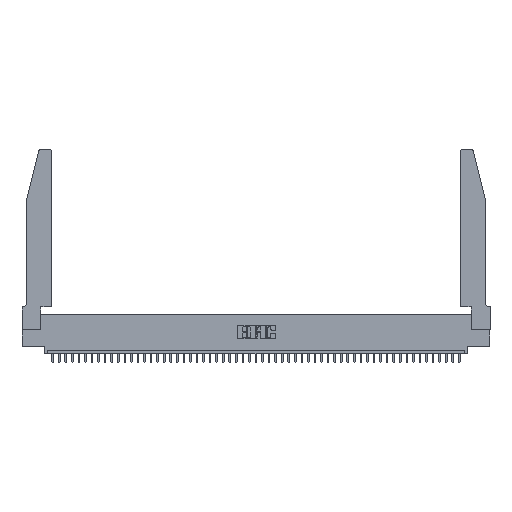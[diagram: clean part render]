
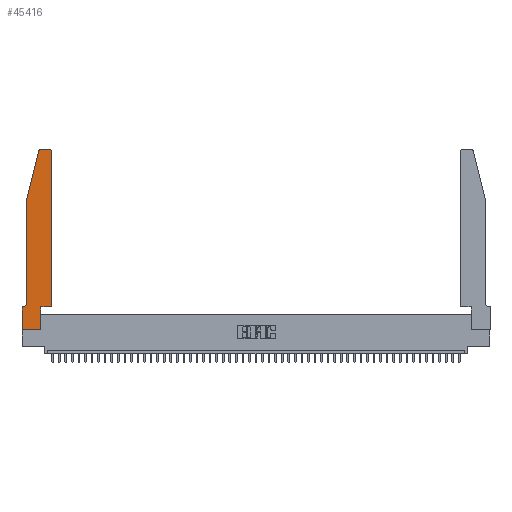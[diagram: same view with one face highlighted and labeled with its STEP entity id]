
A CAD part, top view. The second image highlights one B-rep face of the part: STEP entity #45416.
In plain terms, the highlighted planar face has unit normal (0, 0, 1).
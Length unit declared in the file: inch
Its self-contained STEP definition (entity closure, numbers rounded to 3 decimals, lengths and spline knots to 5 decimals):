
#341 = PLANE ( 'NONE',  #30279 ) ;
#1431 = LINE ( 'NONE', #37344, #19328 ) ;
#1948 = VERTEX_POINT ( 'NONE', #45646 ) ;
#2247 = ORIENTED_EDGE ( 'NONE', *, *, #24732, .T. ) ;
#2251 = DIRECTION ( 'NONE',  ( -1., 0., 0. ) ) ;
#2310 = CARTESIAN_POINT ( 'NONE',  ( 0.284, 2.72, 0.37 ) ) ;
#2726 = VECTOR ( 'NONE', #29254, 39.37008 ) ;
#3358 = AXIS2_PLACEMENT_3D ( 'NONE', #44362, #21430, #2251 ) ;
#3951 = LINE ( 'NONE', #23775, #9359 ) ;
#4026 = CARTESIAN_POINT ( 'NONE',  ( 0., 0.35, 0.37 ) ) ;
#4238 = ORIENTED_EDGE ( 'NONE', *, *, #40683, .T. ) ;
#6506 = VECTOR ( 'NONE', #29017, 39.37008 ) ;
#6556 = LINE ( 'NONE', #21689, #44270 ) ;
#6789 = CARTESIAN_POINT ( 'NONE',  ( 0.2865, 0.35, 0.37 ) ) ;
#6815 = CARTESIAN_POINT ( 'NONE',  ( 0., 0., 0.37 ) ) ;
#7213 = VERTEX_POINT ( 'NONE', #27663 ) ;
#8018 = LINE ( 'NONE', #9886, #2726 ) ;
#9359 = VECTOR ( 'NONE', #40073, 39.37008 ) ;
#9886 = CARTESIAN_POINT ( 'NONE',  ( 0.2865, 0.35, 0.37 ) ) ;
#10471 = DIRECTION ( 'NONE',  ( 1., 0., 0. ) ) ;
#10653 = LINE ( 'NONE', #16750, #6506 ) ;
#10890 = VERTEX_POINT ( 'NONE', #46269 ) ;
#11390 = EDGE_CURVE ( 'NONE', #10890, #7213, #33859, .T. ) ;
#11550 = DIRECTION ( 'NONE',  ( 0., 0., 1. ) ) ;
#11642 = DIRECTION ( 'NONE',  ( 0., 1., 0. ) ) ;
#11790 = EDGE_CURVE ( 'NONE', #43213, #23898, #8018, .T. ) ;
#13609 = VERTEX_POINT ( 'NONE', #44633 ) ;
#13889 = CARTESIAN_POINT ( 'NONE',  ( 0.4205, 2.72, 0.37 ) ) ;
#14196 = ORIENTED_EDGE ( 'NONE', *, *, #23156, .T. ) ;
#15186 = VERTEX_POINT ( 'NONE', #43532 ) ;
#15848 = DIRECTION ( 'NONE',  ( 1., 0., 0. ) ) ;
#15994 = AXIS2_PLACEMENT_3D ( 'NONE', #2310, #32896, #10471 ) ;
#16124 = CARTESIAN_POINT ( 'NONE',  ( 0.0755, 0.42, 0.37 ) ) ;
#16750 = CARTESIAN_POINT ( 'NONE',  ( 0., 0., 0.37 ) ) ;
#16976 = CARTESIAN_POINT ( 'NONE',  ( 0., 0.35, 0.37 ) ) ;
#17239 = EDGE_CURVE ( 'NONE', #40031, #40582, #37702, .T. ) ;
#17250 = EDGE_CURVE ( 'NONE', #15186, #34043, #18529, .T. ) ;
#17297 = LINE ( 'NONE', #45942, #26267 ) ;
#18529 = LINE ( 'NONE', #39431, #23836 ) ;
#19328 = VECTOR ( 'NONE', #41161, 39.37008 ) ;
#20838 = DIRECTION ( 'NONE',  ( 0., 0., 1. ) ) ;
#21008 = ORIENTED_EDGE ( 'NONE', *, *, #23446, .T. ) ;
#21430 = DIRECTION ( 'NONE',  ( 0., 0., -1. ) ) ;
#21513 = DIRECTION ( 'NONE',  ( 0., -1., 0. ) ) ;
#21606 = EDGE_CURVE ( 'NONE', #13609, #25990, #25603, .T. ) ;
#21689 = CARTESIAN_POINT ( 'NONE',  ( 0.2605, 2.75, 0.37 ) ) ;
#23156 = EDGE_CURVE ( 'NONE', #23898, #24640, #3951, .T. ) ;
#23446 = EDGE_CURVE ( 'NONE', #34043, #40031, #29663, .T. ) ;
#23775 = CARTESIAN_POINT ( 'NONE',  ( 0.4505, 0.35, 0.37 ) ) ;
#23836 = VECTOR ( 'NONE', #36988, 39.37008 ) ;
#23898 = VERTEX_POINT ( 'NONE', #6789 ) ;
#24589 = FACE_OUTER_BOUND ( 'NONE', #31035, .T. ) ;
#24640 = VERTEX_POINT ( 'NONE', #45241 ) ;
#24732 = EDGE_CURVE ( 'NONE', #25990, #15186, #1431, .T. ) ;
#24985 = LINE ( 'NONE', #6815, #25575 ) ;
#25575 = VECTOR ( 'NONE', #21513, 39.37008 ) ;
#25603 = CIRCLE ( 'NONE', #15994, 0.03 ) ;
#25990 = VERTEX_POINT ( 'NONE', #43515 ) ;
#26164 = ORIENTED_EDGE ( 'NONE', *, *, #11390, .T. ) ;
#26267 = VECTOR ( 'NONE', #11642, 39.37008 ) ;
#26702 = ORIENTED_EDGE ( 'NONE', *, *, #41178, .T. ) ;
#26908 = ORIENTED_EDGE ( 'NONE', *, *, #17250, .T. ) ;
#27663 = CARTESIAN_POINT ( 'NONE',  ( 0.4205, 2.75, 0.37 ) ) ;
#29017 = DIRECTION ( 'NONE',  ( 1., 0., 0. ) ) ;
#29254 = DIRECTION ( 'NONE',  ( 0., 1., 0. ) ) ;
#29392 = ORIENTED_EDGE ( 'NONE', *, *, #21606, .T. ) ;
#29663 = CIRCLE ( 'NONE', #3358, 0.07 ) ;
#30279 = AXIS2_PLACEMENT_3D ( 'NONE', #4026, #11550, #15848 ) ;
#31035 = EDGE_LOOP ( 'NONE', ( #4238, #29392, #2247, #26908, #21008, #43499, #39993, #26702, #38931, #14196, #33309, #26164 ) ) ;
#31607 = VECTOR ( 'NONE', #32754, 39.37008 ) ;
#32754 = DIRECTION ( 'NONE',  ( -1., 0., 0. ) ) ;
#32896 = DIRECTION ( 'NONE',  ( 0., 0., 1. ) ) ;
#33062 = CARTESIAN_POINT ( 'NONE',  ( 0.0055, 0.35, 0.37 ) ) ;
#33309 = ORIENTED_EDGE ( 'NONE', *, *, #40378, .T. ) ;
#33479 = AXIS2_PLACEMENT_3D ( 'NONE', #13889, #20838, #46283 ) ;
#33859 = CIRCLE ( 'NONE', #33479, 0.03 ) ;
#34043 = VERTEX_POINT ( 'NONE', #16124 ) ;
#36382 = CARTESIAN_POINT ( 'NONE',  ( 0.2865, 0., 0.37 ) ) ;
#36988 = DIRECTION ( 'NONE',  ( 0., -1., 0. ) ) ;
#37344 = CARTESIAN_POINT ( 'NONE',  ( 0.0755, 2., 0.37 ) ) ;
#37702 = LINE ( 'NONE', #42127, #31607 ) ;
#38931 = ORIENTED_EDGE ( 'NONE', *, *, #11790, .T. ) ;
#39431 = CARTESIAN_POINT ( 'NONE',  ( 0.0755, 2., 0.37 ) ) ;
#39993 = ORIENTED_EDGE ( 'NONE', *, *, #47272, .T. ) ;
#40031 = VERTEX_POINT ( 'NONE', #33062 ) ;
#40073 = DIRECTION ( 'NONE',  ( 1., 0., 0. ) ) ;
#40378 = EDGE_CURVE ( 'NONE', #24640, #10890, #17297, .T. ) ;
#40582 = VERTEX_POINT ( 'NONE', #16976 ) ;
#40603 = DIRECTION ( 'NONE',  ( -1., 0., 0. ) ) ;
#40683 = EDGE_CURVE ( 'NONE', #7213, #13609, #6556, .T. ) ;
#41161 = DIRECTION ( 'NONE',  ( -0.239, -0.971, 0. ) ) ;
#41178 = EDGE_CURVE ( 'NONE', #1948, #43213, #10653, .T. ) ;
#42127 = CARTESIAN_POINT ( 'NONE',  ( 0.0755, 0.35, 0.37 ) ) ;
#43213 = VERTEX_POINT ( 'NONE', #36382 ) ;
#43499 = ORIENTED_EDGE ( 'NONE', *, *, #17239, .T. ) ;
#43515 = CARTESIAN_POINT ( 'NONE',  ( 0.25487, 2.72718, 0.37 ) ) ;
#43532 = CARTESIAN_POINT ( 'NONE',  ( 0.0755, 2., 0.37 ) ) ;
#44270 = VECTOR ( 'NONE', #40603, 39.37008 ) ;
#44362 = CARTESIAN_POINT ( 'NONE',  ( 0.0055, 0.42, 0.37 ) ) ;
#44633 = CARTESIAN_POINT ( 'NONE',  ( 0.284, 2.75, 0.37 ) ) ;
#45241 = CARTESIAN_POINT ( 'NONE',  ( 0.4505, 0.35, 0.37 ) ) ;
#45416 = ADVANCED_FACE ( 'NONE', ( #24589 ), #341, .T. ) ;
#45646 = CARTESIAN_POINT ( 'NONE',  ( 0., 0., 0.37 ) ) ;
#45942 = CARTESIAN_POINT ( 'NONE',  ( 0.4505, 0.35, 0.37 ) ) ;
#46269 = CARTESIAN_POINT ( 'NONE',  ( 0.4505, 2.72, 0.37 ) ) ;
#46283 = DIRECTION ( 'NONE',  ( 1., 0., 0. ) ) ;
#47272 = EDGE_CURVE ( 'NONE', #40582, #1948, #24985, .T. ) ;
